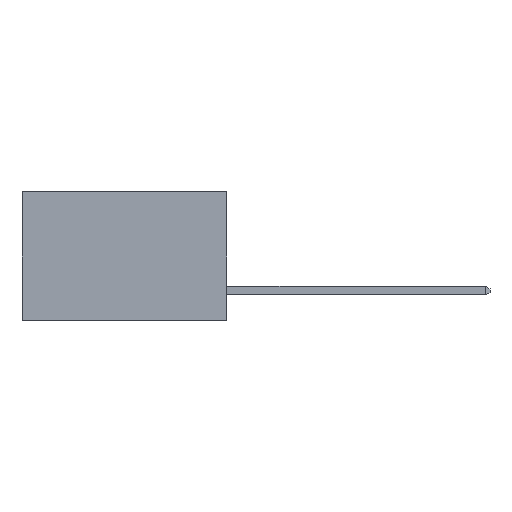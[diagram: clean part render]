
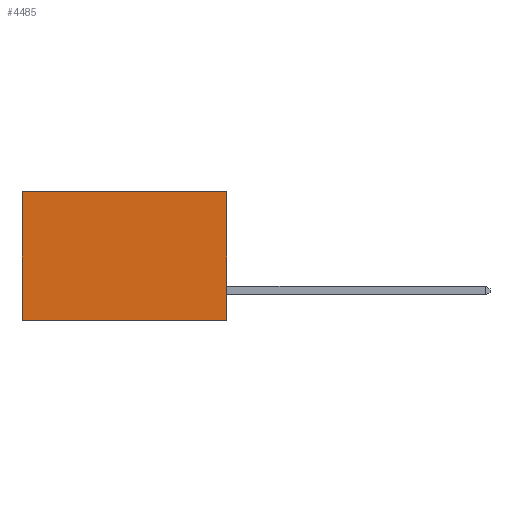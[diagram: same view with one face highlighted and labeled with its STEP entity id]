
A CAD part, left-side view. The second image highlights one B-rep face of the part: STEP entity #4485.
In plain terms, the highlighted planar face has unit normal (-1, 0, 0).
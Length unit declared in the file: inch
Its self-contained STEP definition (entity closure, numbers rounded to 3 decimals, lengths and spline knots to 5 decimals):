
#138 = EDGE_CURVE ( 'NONE', #3554, #2190, #3692, .T. ) ;
#240 = LINE ( 'NONE', #5361, #470 ) ;
#470 = VECTOR ( 'NONE', #5394, 39.37008 ) ;
#486 = FACE_OUTER_BOUND ( 'NONE', #6736, .T. ) ;
#933 = CARTESIAN_POINT ( 'NONE',  ( 0.277, 0., -0.37 ) ) ;
#968 = DIRECTION ( 'NONE',  ( 0., 0., -1. ) ) ;
#1011 = VERTEX_POINT ( 'NONE', #8121 ) ;
#1592 = CARTESIAN_POINT ( 'NONE',  ( 0.277, 0.59, -0.37 ) ) ;
#1640 = DIRECTION ( 'NONE',  ( 0., 0., -1. ) ) ;
#2041 = LINE ( 'NONE', #1592, #5494 ) ;
#2053 = EDGE_CURVE ( 'NONE', #1011, #7510, #2041, .T. ) ;
#2190 = VERTEX_POINT ( 'NONE', #5500 ) ;
#2670 = ORIENTED_EDGE ( 'NONE', *, *, #2053, .T. ) ;
#2883 = ORIENTED_EDGE ( 'NONE', *, *, #5530, .F. ) ;
#3164 = ORIENTED_EDGE ( 'NONE', *, *, #138, .F. ) ;
#3203 = ORIENTED_EDGE ( 'NONE', *, *, #7290, .T. ) ;
#3528 = DIRECTION ( 'NONE',  ( 0., 1., 0. ) ) ;
#3554 = VERTEX_POINT ( 'NONE', #6925 ) ;
#3692 = LINE ( 'NONE', #933, #6881 ) ;
#4485 = ADVANCED_FACE ( 'NONE', ( #486 ), #6222, .F. ) ;
#4511 = VECTOR ( 'NONE', #3528, 39.37008 ) ;
#5361 = CARTESIAN_POINT ( 'NONE',  ( 0.277, 0., -0.37 ) ) ;
#5394 = DIRECTION ( 'NONE',  ( 0., 1., 0. ) ) ;
#5494 = VECTOR ( 'NONE', #1640, 39.37008 ) ;
#5500 = CARTESIAN_POINT ( 'NONE',  ( 0.277, 0., -0.37 ) ) ;
#5530 = EDGE_CURVE ( 'NONE', #2190, #7510, #240, .T. ) ;
#6179 = DIRECTION ( 'NONE',  ( 0., 0., -1. ) ) ;
#6202 = DIRECTION ( 'NONE',  ( 1., 0., 0. ) ) ;
#6212 = CARTESIAN_POINT ( 'NONE',  ( 0.277, 0., -0.37 ) ) ;
#6222 = PLANE ( 'NONE',  #7997 ) ;
#6705 = CARTESIAN_POINT ( 'NONE',  ( 0.277, 0., 0. ) ) ;
#6736 = EDGE_LOOP ( 'NONE', ( #2670, #2883, #3164, #3203 ) ) ;
#6881 = VECTOR ( 'NONE', #968, 39.37008 ) ;
#6925 = CARTESIAN_POINT ( 'NONE',  ( 0.277, 0., 0. ) ) ;
#6985 = CARTESIAN_POINT ( 'NONE',  ( 0.277, 0.59, -0.37 ) ) ;
#7290 = EDGE_CURVE ( 'NONE', #3554, #1011, #8167, .T. ) ;
#7510 = VERTEX_POINT ( 'NONE', #6985 ) ;
#7997 = AXIS2_PLACEMENT_3D ( 'NONE', #6212, #6202, #6179 ) ;
#8121 = CARTESIAN_POINT ( 'NONE',  ( 0.277, 0.59, 0. ) ) ;
#8167 = LINE ( 'NONE', #6705, #4511 ) ;
